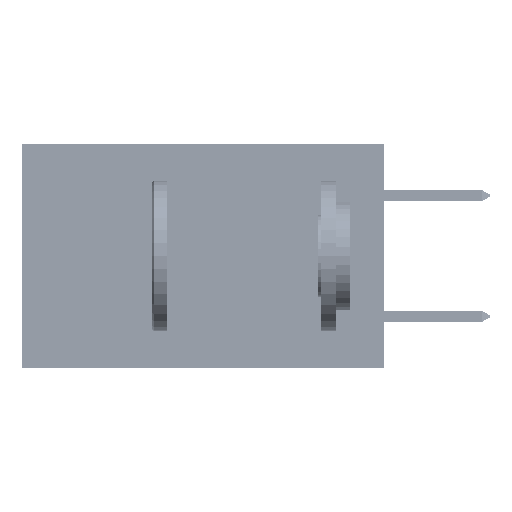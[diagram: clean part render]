
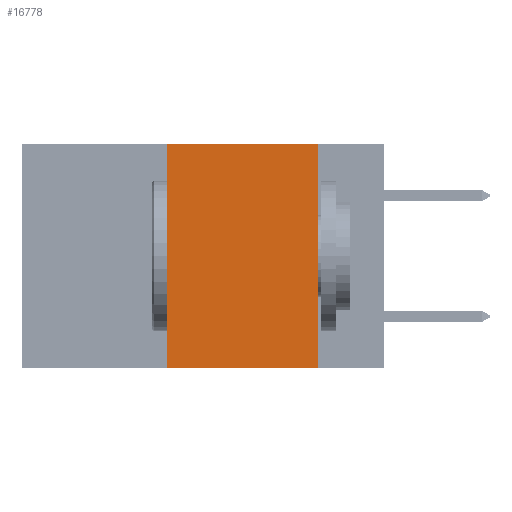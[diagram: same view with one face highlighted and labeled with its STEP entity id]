
A CAD part, left-side view. The second image highlights one B-rep face of the part: STEP entity #16778.
In plain terms, the highlighted planar face has unit normal (-1, 0, 0).
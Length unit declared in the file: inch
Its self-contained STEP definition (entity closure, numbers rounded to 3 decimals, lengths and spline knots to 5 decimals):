
#1034 = EDGE_LOOP ( 'NONE', ( #18995, #23329, #9312, #8770 ) ) ;
#7867 = CARTESIAN_POINT ( 'NONE',  ( 0., 0.36, 0. ) ) ;
#8770 = ORIENTED_EDGE ( 'NONE', *, *, #39654, .T. ) ;
#8896 = CARTESIAN_POINT ( 'NONE',  ( 0., 0.11, 0. ) ) ;
#9312 = ORIENTED_EDGE ( 'NONE', *, *, #38840, .F. ) ;
#10165 = VERTEX_POINT ( 'NONE', #7867 ) ;
#12062 = AXIS2_PLACEMENT_3D ( 'NONE', #39124, #21199, #46523 ) ;
#14438 = LINE ( 'NONE', #17683, #21791 ) ;
#15768 = LINE ( 'NONE', #31549, #24254 ) ;
#16013 = EDGE_CURVE ( 'NONE', #17834, #29948, #15768, .T. ) ;
#16778 = ADVANCED_FACE ( 'NONE', ( #19046 ), #42883, .F. ) ;
#17339 = VECTOR ( 'NONE', #27228, 39.37008 ) ;
#17683 = CARTESIAN_POINT ( 'NONE',  ( 0., 0.6, -0.37 ) ) ;
#17834 = VERTEX_POINT ( 'NONE', #8896 ) ;
#18995 = ORIENTED_EDGE ( 'NONE', *, *, #16013, .F. ) ;
#19046 = FACE_OUTER_BOUND ( 'NONE', #1034, .T. ) ;
#19752 = CARTESIAN_POINT ( 'NONE',  ( 0., 0.36, 0. ) ) ;
#20429 = VECTOR ( 'NONE', #39091, 39.37008 ) ;
#20771 = DIRECTION ( 'NONE',  ( 0., 0., -1. ) ) ;
#21199 = DIRECTION ( 'NONE',  ( 1., 0., 0. ) ) ;
#21301 = DIRECTION ( 'NONE',  ( 0., -1., 0. ) ) ;
#21791 = VECTOR ( 'NONE', #21301, 39.37008 ) ;
#22653 = VERTEX_POINT ( 'NONE', #27398 ) ;
#23329 = ORIENTED_EDGE ( 'NONE', *, *, #35945, .F. ) ;
#24254 = VECTOR ( 'NONE', #20771, 39.37008 ) ;
#27228 = DIRECTION ( 'NONE',  ( 0., 0., 1. ) ) ;
#27398 = CARTESIAN_POINT ( 'NONE',  ( 0., 0.36, -0.37 ) ) ;
#29225 = LINE ( 'NONE', #19752, #17339 ) ;
#29948 = VERTEX_POINT ( 'NONE', #33658 ) ;
#30069 = LINE ( 'NONE', #31797, #20429 ) ;
#31549 = CARTESIAN_POINT ( 'NONE',  ( 0., 0.11, 0. ) ) ;
#31797 = CARTESIAN_POINT ( 'NONE',  ( 0., 0.6, 0. ) ) ;
#33658 = CARTESIAN_POINT ( 'NONE',  ( 0., 0.11, -0.37 ) ) ;
#35945 = EDGE_CURVE ( 'NONE', #10165, #17834, #30069, .T. ) ;
#38840 = EDGE_CURVE ( 'NONE', #22653, #10165, #29225, .T. ) ;
#39091 = DIRECTION ( 'NONE',  ( 0., -1., 0. ) ) ;
#39124 = CARTESIAN_POINT ( 'NONE',  ( 0., 0.6, 0. ) ) ;
#39654 = EDGE_CURVE ( 'NONE', #22653, #29948, #14438, .T. ) ;
#42883 = PLANE ( 'NONE',  #12062 ) ;
#46523 = DIRECTION ( 'NONE',  ( 0., 0., -1. ) ) ;
